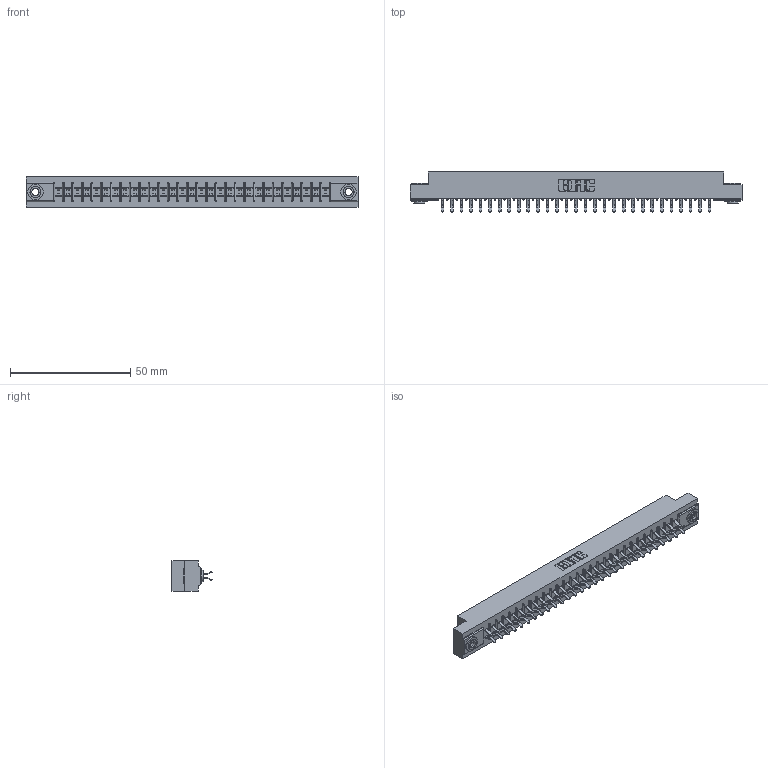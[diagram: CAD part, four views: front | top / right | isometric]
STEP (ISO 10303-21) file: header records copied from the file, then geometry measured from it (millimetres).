
FILE_DESCRIPTION (( 'STEP AP203' ), '1' );
FILE_NAME ('355-058-556-203.STEP', '2019-09-12T13:31:28', ( '' ), ( '' ), 'SwSTEP 2.0', 'SolidWorks 2016', '' );
FILE_SCHEMA (( 'CONFIG_CONTROL_DESIGN' ));
Length unit declared in the file: inch
Products named in the file (4): 345-250-002_345-250-002-102; 355-058-556-203; 305-290-001_556; 305 Part_.156 Dia
Assembly tree (61 placements, depth 2):
  355-058-556-203
    305 Part_.156 Dia
    305-290-001_556  x58
    345-250-002_345-250-002-102  x2
Bounding box: 137.92 x 16.64 x 12.7 mm (x, y, z)
Volume: 14299.1 mm3; surface area: 18170.6 mm2
Topology: 61 solids, 61 shells, 3416 faces, 9795 edges, 6370 vertices
Faces by surface type: plane 1890, cylinder 1402, sphere 116, cone 8
Entity records: 34269 total; most frequent: CARTESIAN_POINT 5654, ORIENTED_EDGE 5602, DIRECTION 5499, EDGE_CURVE 2801, VECTOR 2237, LINE 2237, VERTEX_POINT 1786, AXIS2_PLACEMENT_3D 1631
